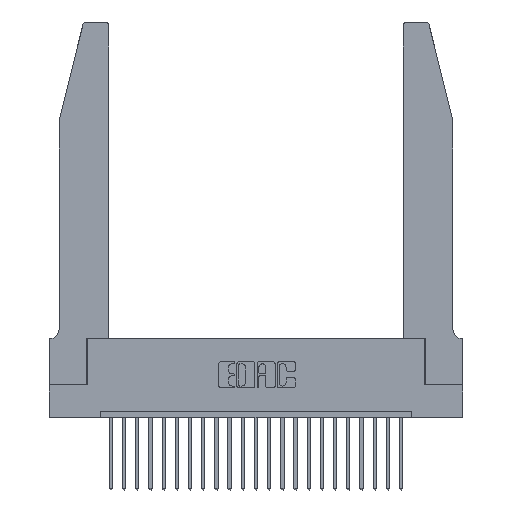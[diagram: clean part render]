
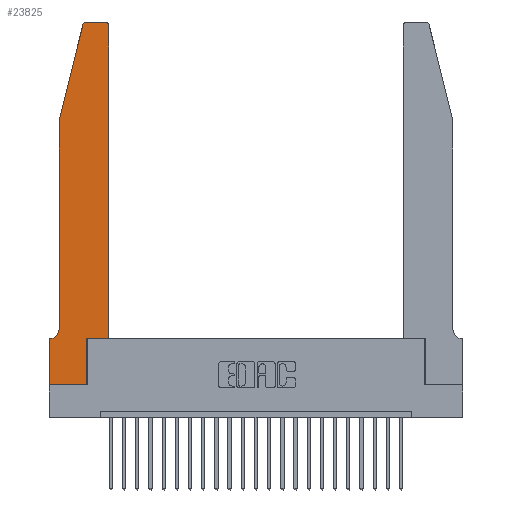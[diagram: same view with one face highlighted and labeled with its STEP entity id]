
A CAD part, top view. The second image highlights one B-rep face of the part: STEP entity #23825.
In plain terms, the highlighted planar face has unit normal (0, 0, 1).
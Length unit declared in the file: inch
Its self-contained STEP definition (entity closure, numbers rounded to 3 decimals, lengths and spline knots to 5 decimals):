
#250 = EDGE_CURVE ( 'NONE', #6781, #736, #2029, .T. ) ;
#316 = EDGE_CURVE ( 'NONE', #8715, #6781, #17799, .T. ) ;
#325 = AXIS2_PLACEMENT_3D ( 'NONE', #18995, #13751, #7995 ) ;
#443 = LINE ( 'NONE', #13227, #16153 ) ;
#562 = VERTEX_POINT ( 'NONE', #13213 ) ;
#736 = VERTEX_POINT ( 'NONE', #2820 ) ;
#937 = VECTOR ( 'NONE', #8651, 39.37008 ) ;
#989 = LINE ( 'NONE', #17233, #15507 ) ;
#1198 = ORIENTED_EDGE ( 'NONE', *, *, #22934, .T. ) ;
#1350 = PLANE ( 'NONE',  #14328 ) ;
#1424 = FACE_OUTER_BOUND ( 'NONE', #16136, .T. ) ;
#1739 = ORIENTED_EDGE ( 'NONE', *, *, #316, .T. ) ;
#1779 = DIRECTION ( 'NONE',  ( 0., 1., 0. ) ) ;
#2029 = LINE ( 'NONE', #14120, #12469 ) ;
#2580 = CARTESIAN_POINT ( 'NONE',  ( 0.2865, 0., 0.37 ) ) ;
#2587 = CARTESIAN_POINT ( 'NONE',  ( 0., 0.35, 0.37 ) ) ;
#2820 = CARTESIAN_POINT ( 'NONE',  ( 0.0755, 0.42, 0.37 ) ) ;
#2846 = DIRECTION ( 'NONE',  ( -0.239, -0.971, 0. ) ) ;
#2965 = VECTOR ( 'NONE', #2846, 39.37008 ) ;
#3018 = EDGE_CURVE ( 'NONE', #12632, #14125, #20299, .T. ) ;
#3076 = AXIS2_PLACEMENT_3D ( 'NONE', #11259, #21033, #20937 ) ;
#3090 = CIRCLE ( 'NONE', #8561, 0.07 ) ;
#3213 = ORIENTED_EDGE ( 'NONE', *, *, #22005, .T. ) ;
#3397 = VERTEX_POINT ( 'NONE', #15329 ) ;
#3420 = EDGE_CURVE ( 'NONE', #3397, #16219, #989, .T. ) ;
#3558 = CARTESIAN_POINT ( 'NONE',  ( 0.4505, 0.35, 0.37 ) ) ;
#4100 = CARTESIAN_POINT ( 'NONE',  ( 0.0755, 2., 0.37 ) ) ;
#4336 = DIRECTION ( 'NONE',  ( 0., 0., -1. ) ) ;
#4425 = DIRECTION ( 'NONE',  ( -1., 0., 0. ) ) ;
#4515 = CARTESIAN_POINT ( 'NONE',  ( 0., 0.35, 0.37 ) ) ;
#5128 = LINE ( 'NONE', #20059, #937 ) ;
#5399 = CIRCLE ( 'NONE', #325, 0.03 ) ;
#5654 = VECTOR ( 'NONE', #20188, 39.37008 ) ;
#5708 = CARTESIAN_POINT ( 'NONE',  ( 0.4505, 0.35, 0.37 ) ) ;
#5992 = ORIENTED_EDGE ( 'NONE', *, *, #3420, .T. ) ;
#6781 = VERTEX_POINT ( 'NONE', #4100 ) ;
#6906 = DIRECTION ( 'NONE',  ( 0., 0., 1. ) ) ;
#7995 = DIRECTION ( 'NONE',  ( 1., 0., 0. ) ) ;
#8139 = CARTESIAN_POINT ( 'NONE',  ( 0., 0., 0.37 ) ) ;
#8561 = AXIS2_PLACEMENT_3D ( 'NONE', #17519, #4336, #4425 ) ;
#8651 = DIRECTION ( 'NONE',  ( -1., 0., 0. ) ) ;
#8715 = VERTEX_POINT ( 'NONE', #16318 ) ;
#8940 = ORIENTED_EDGE ( 'NONE', *, *, #12753, .T. ) ;
#9107 = CIRCLE ( 'NONE', #3076, 0.03 ) ;
#9336 = VERTEX_POINT ( 'NONE', #24476 ) ;
#9440 = DIRECTION ( 'NONE',  ( 0., -1., 0. ) ) ;
#9447 = VERTEX_POINT ( 'NONE', #15135 ) ;
#10124 = LINE ( 'NONE', #18213, #5654 ) ;
#10349 = DIRECTION ( 'NONE',  ( 0., -1., 0. ) ) ;
#10638 = VECTOR ( 'NONE', #15211, 39.37008 ) ;
#10791 = EDGE_CURVE ( 'NONE', #19964, #9336, #21892, .T. ) ;
#11004 = VECTOR ( 'NONE', #14936, 39.37008 ) ;
#11259 = CARTESIAN_POINT ( 'NONE',  ( 0.4205, 2.72, 0.37 ) ) ;
#12469 = VECTOR ( 'NONE', #10349, 39.37008 ) ;
#12552 = CARTESIAN_POINT ( 'NONE',  ( 0.0755, 2., 0.37 ) ) ;
#12632 = VERTEX_POINT ( 'NONE', #2580 ) ;
#12753 = EDGE_CURVE ( 'NONE', #9447, #8715, #5399, .T. ) ;
#13213 = CARTESIAN_POINT ( 'NONE',  ( 0.4205, 2.75, 0.37 ) ) ;
#13227 = CARTESIAN_POINT ( 'NONE',  ( 0., 0., 0.37 ) ) ;
#13751 = DIRECTION ( 'NONE',  ( 0., 0., 1. ) ) ;
#14120 = CARTESIAN_POINT ( 'NONE',  ( 0.0755, 2., 0.37 ) ) ;
#14125 = VERTEX_POINT ( 'NONE', #24092 ) ;
#14328 = AXIS2_PLACEMENT_3D ( 'NONE', #4515, #6906, #20544 ) ;
#14829 = LINE ( 'NONE', #16608, #11004 ) ;
#14888 = ORIENTED_EDGE ( 'NONE', *, *, #3018, .T. ) ;
#14936 = DIRECTION ( 'NONE',  ( 1., 0., 0. ) ) ;
#15135 = CARTESIAN_POINT ( 'NONE',  ( 0.284, 2.75, 0.37 ) ) ;
#15211 = DIRECTION ( 'NONE',  ( 0., 1., 0. ) ) ;
#15329 = CARTESIAN_POINT ( 'NONE',  ( 0.0055, 0.35, 0.37 ) ) ;
#15507 = VECTOR ( 'NONE', #19172, 39.37008 ) ;
#15603 = EDGE_CURVE ( 'NONE', #9336, #562, #9107, .T. ) ;
#16136 = EDGE_LOOP ( 'NONE', ( #3213, #8940, #1739, #16181, #20849, #5992, #18899, #18971, #14888, #1198, #16466, #24594 ) ) ;
#16153 = VECTOR ( 'NONE', #9440, 39.37008 ) ;
#16181 = ORIENTED_EDGE ( 'NONE', *, *, #250, .T. ) ;
#16219 = VERTEX_POINT ( 'NONE', #2587 ) ;
#16318 = CARTESIAN_POINT ( 'NONE',  ( 0.25487, 2.72718, 0.37 ) ) ;
#16466 = ORIENTED_EDGE ( 'NONE', *, *, #10791, .T. ) ;
#16608 = CARTESIAN_POINT ( 'NONE',  ( 0.4505, 0.35, 0.37 ) ) ;
#17233 = CARTESIAN_POINT ( 'NONE',  ( 0.0755, 0.35, 0.37 ) ) ;
#17287 = EDGE_CURVE ( 'NONE', #736, #3397, #3090, .T. ) ;
#17519 = CARTESIAN_POINT ( 'NONE',  ( 0.0055, 0.42, 0.37 ) ) ;
#17799 = LINE ( 'NONE', #12552, #2965 ) ;
#18213 = CARTESIAN_POINT ( 'NONE',  ( 0., 0., 0.37 ) ) ;
#18225 = EDGE_CURVE ( 'NONE', #16219, #20587, #443, .T. ) ;
#18885 = CARTESIAN_POINT ( 'NONE',  ( 0.2865, 0.35, 0.37 ) ) ;
#18899 = ORIENTED_EDGE ( 'NONE', *, *, #18225, .T. ) ;
#18971 = ORIENTED_EDGE ( 'NONE', *, *, #22745, .T. ) ;
#18995 = CARTESIAN_POINT ( 'NONE',  ( 0.284, 2.72, 0.37 ) ) ;
#19172 = DIRECTION ( 'NONE',  ( -1., 0., 0. ) ) ;
#19964 = VERTEX_POINT ( 'NONE', #3558 ) ;
#20059 = CARTESIAN_POINT ( 'NONE',  ( 0.2605, 2.75, 0.37 ) ) ;
#20188 = DIRECTION ( 'NONE',  ( 1., 0., 0. ) ) ;
#20299 = LINE ( 'NONE', #18885, #22720 ) ;
#20544 = DIRECTION ( 'NONE',  ( 1., 0., 0. ) ) ;
#20587 = VERTEX_POINT ( 'NONE', #8139 ) ;
#20849 = ORIENTED_EDGE ( 'NONE', *, *, #17287, .T. ) ;
#20937 = DIRECTION ( 'NONE',  ( 1., 0., 0. ) ) ;
#21033 = DIRECTION ( 'NONE',  ( 0., 0., 1. ) ) ;
#21892 = LINE ( 'NONE', #5708, #10638 ) ;
#22005 = EDGE_CURVE ( 'NONE', #562, #9447, #5128, .T. ) ;
#22720 = VECTOR ( 'NONE', #1779, 39.37008 ) ;
#22745 = EDGE_CURVE ( 'NONE', #20587, #12632, #10124, .T. ) ;
#22934 = EDGE_CURVE ( 'NONE', #14125, #19964, #14829, .T. ) ;
#23825 = ADVANCED_FACE ( 'NONE', ( #1424 ), #1350, .T. ) ;
#24092 = CARTESIAN_POINT ( 'NONE',  ( 0.2865, 0.35, 0.37 ) ) ;
#24476 = CARTESIAN_POINT ( 'NONE',  ( 0.4505, 2.72, 0.37 ) ) ;
#24594 = ORIENTED_EDGE ( 'NONE', *, *, #15603, .T. ) ;
